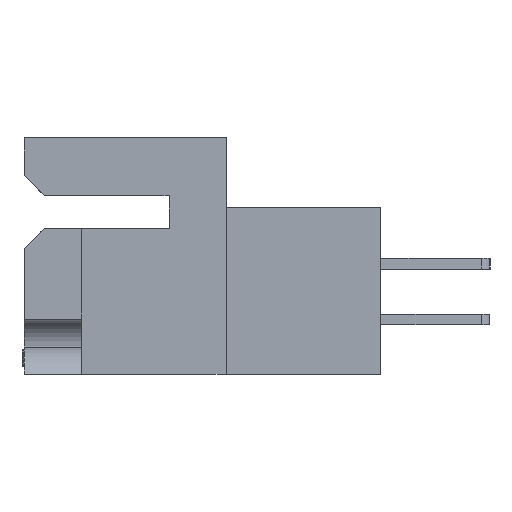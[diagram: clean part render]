
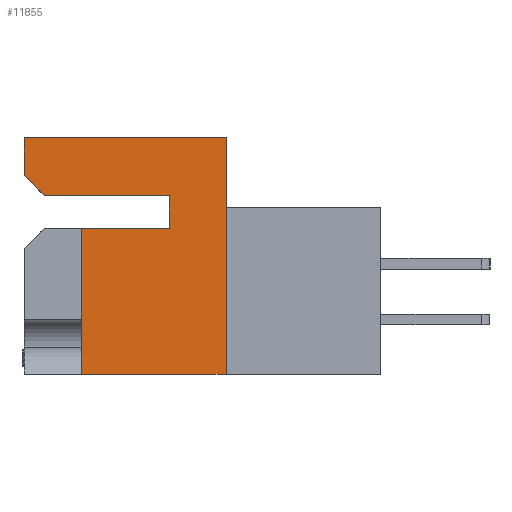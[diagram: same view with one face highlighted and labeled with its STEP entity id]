
A CAD part, left-side view. The second image highlights one B-rep face of the part: STEP entity #11855.
In plain terms, the highlighted planar face has unit normal (-1, 0, 0).
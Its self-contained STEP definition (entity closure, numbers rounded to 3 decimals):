
#617 = CARTESIAN_POINT ( 'NONE',  ( 0., 0., -5.182 ) ) ;
#698 = EDGE_CURVE ( 'NONE', #3389, #13289, #8863, .T. ) ;
#1093 = CARTESIAN_POINT ( 'NONE',  ( 0., 0., 0. ) ) ;
#1290 = DIRECTION ( 'NONE',  ( 0., 0., -1. ) ) ;
#1427 = VERTEX_POINT ( 'NONE', #4176 ) ;
#1465 = VERTEX_POINT ( 'NONE', #11317 ) ;
#1925 = CARTESIAN_POINT ( 'NONE',  ( 0., 11.506, 0. ) ) ;
#2028 = CARTESIAN_POINT ( 'NONE',  ( 0., 8.255, -5.182 ) ) ;
#2638 = PLANE ( 'NONE',  #21514 ) ;
#3025 = VECTOR ( 'NONE', #18437, 1000. ) ;
#3063 = VECTOR ( 'NONE', #29435, 1000. ) ;
#3150 = VERTEX_POINT ( 'NONE', #2028 ) ;
#3181 = VERTEX_POINT ( 'NONE', #1925 ) ;
#3315 = LINE ( 'NONE', #28595, #8727 ) ;
#3389 = VERTEX_POINT ( 'NONE', #10289 ) ;
#4176 = CARTESIAN_POINT ( 'NONE',  ( 0., 0., 0. ) ) ;
#4602 = DIRECTION ( 'NONE',  ( 0., -0.707, -0.707 ) ) ;
#4754 = EDGE_CURVE ( 'NONE', #13289, #3150, #3315, .T. ) ;
#4837 = CARTESIAN_POINT ( 'NONE',  ( 0., 0., -3.302 ) ) ;
#5879 = LINE ( 'NONE', #617, #17419 ) ;
#5904 = VERTEX_POINT ( 'NONE', #24281 ) ;
#6055 = ORIENTED_EDGE ( 'NONE', *, *, #698, .F. ) ;
#6686 = DIRECTION ( 'NONE',  ( 0., 0., 1. ) ) ;
#7320 = DIRECTION ( 'NONE',  ( 0., 1., 0. ) ) ;
#7748 = LINE ( 'NONE', #24511, #3063 ) ;
#7799 = CARTESIAN_POINT ( 'NONE',  ( 0., 11.506, -2.159 ) ) ;
#8305 = EDGE_LOOP ( 'NONE', ( #6055, #11329, #17770, #29862, #24881, #9509, #10905, #19586, #26572 ) ) ;
#8462 = VECTOR ( 'NONE', #6686, 1000. ) ;
#8727 = VECTOR ( 'NONE', #28308, 1000. ) ;
#8863 = LINE ( 'NONE', #23865, #12794 ) ;
#9509 = ORIENTED_EDGE ( 'NONE', *, *, #22054, .F. ) ;
#9609 = CARTESIAN_POINT ( 'NONE',  ( 0., 11.506, -13.487 ) ) ;
#10289 = CARTESIAN_POINT ( 'NONE',  ( 0., 0., -13.487 ) ) ;
#10905 = ORIENTED_EDGE ( 'NONE', *, *, #28432, .F. ) ;
#11317 = CARTESIAN_POINT ( 'NONE',  ( 0., 10.363, -3.302 ) ) ;
#11329 = ORIENTED_EDGE ( 'NONE', *, *, #26843, .F. ) ;
#11747 = FACE_OUTER_BOUND ( 'NONE', #8305, .T. ) ;
#11855 = ADVANCED_FACE ( 'NONE', ( #11747 ), #2638, .F. ) ;
#12619 = DIRECTION ( 'NONE',  ( 0., -1., 0. ) ) ;
#12794 = VECTOR ( 'NONE', #7320, 1000. ) ;
#13289 = VERTEX_POINT ( 'NONE', #16063 ) ;
#13937 = LINE ( 'NONE', #17741, #27687 ) ;
#14411 = CARTESIAN_POINT ( 'NONE',  ( 0., 11.506, 0. ) ) ;
#14761 = VERTEX_POINT ( 'NONE', #7799 ) ;
#16063 = CARTESIAN_POINT ( 'NONE',  ( 0., 8.255, -13.487 ) ) ;
#17038 = DIRECTION ( 'NONE',  ( 1., 0., 0. ) ) ;
#17374 = VECTOR ( 'NONE', #4602, 1000. ) ;
#17419 = VECTOR ( 'NONE', #12619, 1000. ) ;
#17741 = CARTESIAN_POINT ( 'NONE',  ( 0., 0., 0. ) ) ;
#17770 = ORIENTED_EDGE ( 'NONE', *, *, #23850, .F. ) ;
#18437 = DIRECTION ( 'NONE',  ( 0., 1., 0. ) ) ;
#18513 = CARTESIAN_POINT ( 'NONE',  ( 0., 3.251, -3.302 ) ) ;
#19586 = ORIENTED_EDGE ( 'NONE', *, *, #29450, .F. ) ;
#20248 = CARTESIAN_POINT ( 'NONE',  ( 0., 10.363, -3.302 ) ) ;
#21436 = LINE ( 'NONE', #4837, #3025 ) ;
#21471 = EDGE_CURVE ( 'NONE', #14761, #3181, #27590, .T. ) ;
#21514 = AXIS2_PLACEMENT_3D ( 'NONE', #1093, #17038, #21907 ) ;
#21907 = DIRECTION ( 'NONE',  ( 0., 0., -1. ) ) ;
#22054 = EDGE_CURVE ( 'NONE', #24850, #1465, #21436, .T. ) ;
#23132 = EDGE_CURVE ( 'NONE', #14761, #1465, #23540, .T. ) ;
#23540 = LINE ( 'NONE', #20248, #17374 ) ;
#23850 = EDGE_CURVE ( 'NONE', #3181, #1427, #25642, .T. ) ;
#23865 = CARTESIAN_POINT ( 'NONE',  ( 0., -8.814, -13.487 ) ) ;
#24281 = CARTESIAN_POINT ( 'NONE',  ( 0., 3.251, -5.182 ) ) ;
#24511 = CARTESIAN_POINT ( 'NONE',  ( 0., 3.251, -5.182 ) ) ;
#24850 = VERTEX_POINT ( 'NONE', #18513 ) ;
#24881 = ORIENTED_EDGE ( 'NONE', *, *, #23132, .T. ) ;
#24930 = VECTOR ( 'NONE', #28262, 1000. ) ;
#25642 = LINE ( 'NONE', #14411, #24930 ) ;
#26572 = ORIENTED_EDGE ( 'NONE', *, *, #4754, .F. ) ;
#26843 = EDGE_CURVE ( 'NONE', #1427, #3389, #13937, .T. ) ;
#27590 = LINE ( 'NONE', #9609, #8462 ) ;
#27687 = VECTOR ( 'NONE', #1290, 1000. ) ;
#28262 = DIRECTION ( 'NONE',  ( 0., -1., 0. ) ) ;
#28308 = DIRECTION ( 'NONE',  ( 0., 0., 1. ) ) ;
#28432 = EDGE_CURVE ( 'NONE', #5904, #24850, #7748, .T. ) ;
#28595 = CARTESIAN_POINT ( 'NONE',  ( 0., 8.255, -5.182 ) ) ;
#29435 = DIRECTION ( 'NONE',  ( 0., 0., 1. ) ) ;
#29450 = EDGE_CURVE ( 'NONE', #3150, #5904, #5879, .T. ) ;
#29862 = ORIENTED_EDGE ( 'NONE', *, *, #21471, .F. ) ;
